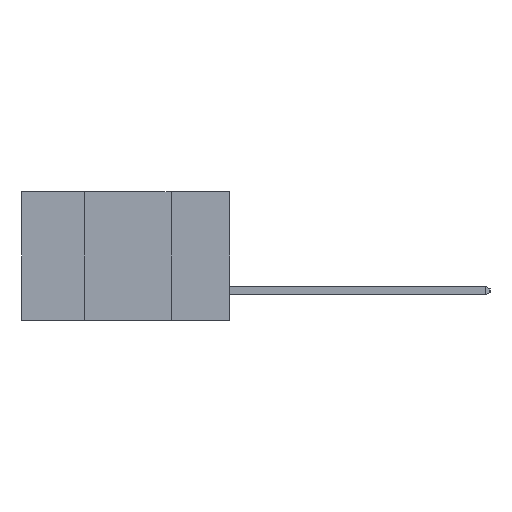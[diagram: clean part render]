
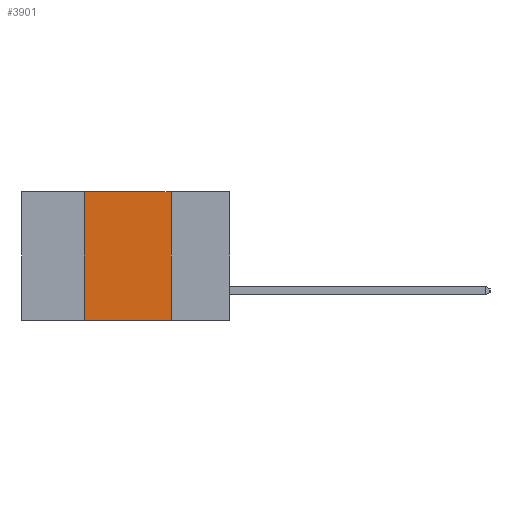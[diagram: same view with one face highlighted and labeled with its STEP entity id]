
A CAD part, left-side view. The second image highlights one B-rep face of the part: STEP entity #3901.
In plain terms, the highlighted planar face has unit normal (-1, 0, 0).
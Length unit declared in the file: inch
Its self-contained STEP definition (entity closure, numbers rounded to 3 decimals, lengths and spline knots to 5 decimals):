
#435 = VECTOR ( 'NONE', #18569, 39.37008 ) ;
#1794 = CARTESIAN_POINT ( 'NONE',  ( 0., 0.42, 0. ) ) ;
#3190 = VECTOR ( 'NONE', #3822, 39.37008 ) ;
#3822 = DIRECTION ( 'NONE',  ( 0., 0., 1. ) ) ;
#3901 = ADVANCED_FACE ( 'NONE', ( #4574 ), #4132, .F. ) ;
#4132 = PLANE ( 'NONE',  #15025 ) ;
#4574 = FACE_OUTER_BOUND ( 'NONE', #6823, .T. ) ;
#4762 = DIRECTION ( 'NONE',  ( 0., -1., 0. ) ) ;
#6823 = EDGE_LOOP ( 'NONE', ( #9211, #9268, #9544, #9571 ) ) ;
#7107 = CARTESIAN_POINT ( 'NONE',  ( 0., 0.17, 0. ) ) ;
#8641 = CARTESIAN_POINT ( 'NONE',  ( 0., 0.42, -0.37 ) ) ;
#9211 = ORIENTED_EDGE ( 'NONE', *, *, #10748, .F. ) ;
#9268 = ORIENTED_EDGE ( 'NONE', *, *, #13122, .F. ) ;
#9544 = ORIENTED_EDGE ( 'NONE', *, *, #12120, .F. ) ;
#9571 = ORIENTED_EDGE ( 'NONE', *, *, #16218, .T. ) ;
#10748 = EDGE_CURVE ( 'NONE', #24057, #20003, #21163, .T. ) ;
#12120 = EDGE_CURVE ( 'NONE', #19443, #14236, #24899, .T. ) ;
#13122 = EDGE_CURVE ( 'NONE', #14236, #24057, #16810, .T. ) ;
#14236 = VERTEX_POINT ( 'NONE', #20051 ) ;
#15025 = AXIS2_PLACEMENT_3D ( 'NONE', #24743, #23448, #23359 ) ;
#15772 = VECTOR ( 'NONE', #24093, 39.37008 ) ;
#16218 = EDGE_CURVE ( 'NONE', #19443, #20003, #19192, .T. ) ;
#16516 = CARTESIAN_POINT ( 'NONE',  ( 0., 0.17, -0.37 ) ) ;
#16571 = CARTESIAN_POINT ( 'NONE',  ( 0., 0.6, 0. ) ) ;
#16810 = LINE ( 'NONE', #16571, #435 ) ;
#18569 = DIRECTION ( 'NONE',  ( 0., -1., 0. ) ) ;
#18996 = CARTESIAN_POINT ( 'NONE',  ( 0., 0.6, -0.37 ) ) ;
#19192 = LINE ( 'NONE', #18996, #23949 ) ;
#19443 = VERTEX_POINT ( 'NONE', #8641 ) ;
#20003 = VERTEX_POINT ( 'NONE', #16516 ) ;
#20051 = CARTESIAN_POINT ( 'NONE',  ( 0., 0.42, 0. ) ) ;
#21163 = LINE ( 'NONE', #26100, #15772 ) ;
#23359 = DIRECTION ( 'NONE',  ( 0., 0., -1. ) ) ;
#23448 = DIRECTION ( 'NONE',  ( 1., 0., 0. ) ) ;
#23949 = VECTOR ( 'NONE', #4762, 39.37008 ) ;
#24057 = VERTEX_POINT ( 'NONE', #7107 ) ;
#24093 = DIRECTION ( 'NONE',  ( 0., 0., -1. ) ) ;
#24743 = CARTESIAN_POINT ( 'NONE',  ( 0., 0.6, 0. ) ) ;
#24899 = LINE ( 'NONE', #1794, #3190 ) ;
#26100 = CARTESIAN_POINT ( 'NONE',  ( 0., 0.17, 0. ) ) ;
